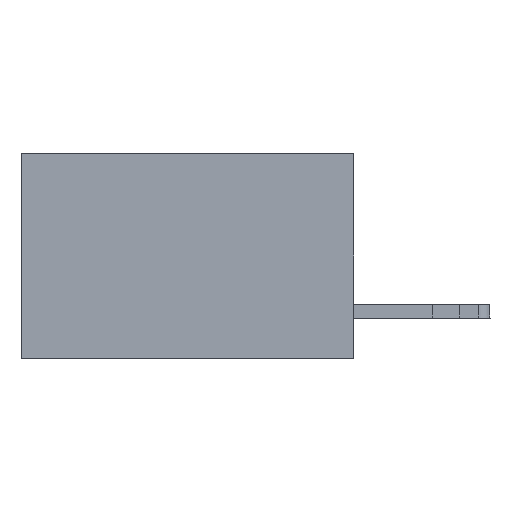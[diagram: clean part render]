
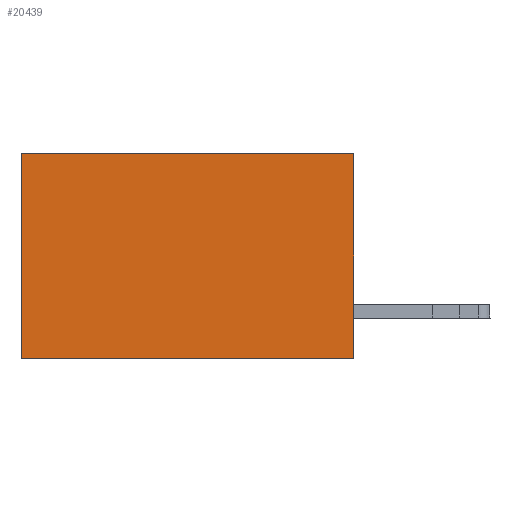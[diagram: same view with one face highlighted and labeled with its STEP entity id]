
A CAD part, left-side view. The second image highlights one B-rep face of the part: STEP entity #20439.
In plain terms, the highlighted planar face has unit normal (-1, 0, 0).
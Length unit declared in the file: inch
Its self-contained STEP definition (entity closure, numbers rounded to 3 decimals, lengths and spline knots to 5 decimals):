
#616 = ORIENTED_EDGE ( 'NONE', *, *, #26338, .T. ) ;
#1786 = VECTOR ( 'NONE', #6886, 39.37008 ) ;
#1950 = VERTEX_POINT ( 'NONE', #5260 ) ;
#3957 = LINE ( 'NONE', #32492, #34746 ) ;
#4269 = DIRECTION ( 'NONE',  ( 0., 1., 0. ) ) ;
#5260 = CARTESIAN_POINT ( 'NONE',  ( 0.2875, 0.6, 0. ) ) ;
#6886 = DIRECTION ( 'NONE',  ( 0., 0., -1. ) ) ;
#7437 = ORIENTED_EDGE ( 'NONE', *, *, #35931, .F. ) ;
#7439 = LINE ( 'NONE', #18447, #1786 ) ;
#8702 = DIRECTION ( 'NONE',  ( 0., 0., -1. ) ) ;
#9938 = VERTEX_POINT ( 'NONE', #36319 ) ;
#10741 = ORIENTED_EDGE ( 'NONE', *, *, #20627, .F. ) ;
#11693 = FACE_OUTER_BOUND ( 'NONE', #29390, .T. ) ;
#11878 = DIRECTION ( 'NONE',  ( 1., 0., 0. ) ) ;
#14487 = CARTESIAN_POINT ( 'NONE',  ( 0.2875, 0., 0. ) ) ;
#14861 = EDGE_CURVE ( 'NONE', #1950, #28969, #7439, .T. ) ;
#15591 = LINE ( 'NONE', #35168, #26474 ) ;
#18447 = CARTESIAN_POINT ( 'NONE',  ( 0.2875, 0.6, 0. ) ) ;
#19942 = PLANE ( 'NONE',  #33562 ) ;
#20439 = ADVANCED_FACE ( 'NONE', ( #11693 ), #19942, .F. ) ;
#20627 = EDGE_CURVE ( 'NONE', #9938, #33087, #15591, .T. ) ;
#21245 = CARTESIAN_POINT ( 'NONE',  ( 0.2875, 0., -0.37 ) ) ;
#21685 = DIRECTION ( 'NONE',  ( 0., 1., 0. ) ) ;
#23055 = CARTESIAN_POINT ( 'NONE',  ( 0.2875, 0., -0.37 ) ) ;
#26338 = EDGE_CURVE ( 'NONE', #9938, #1950, #3957, .T. ) ;
#26474 = VECTOR ( 'NONE', #29604, 39.37008 ) ;
#26479 = VECTOR ( 'NONE', #4269, 39.37008 ) ;
#28969 = VERTEX_POINT ( 'NONE', #34351 ) ;
#29390 = EDGE_LOOP ( 'NONE', ( #35006, #7437, #10741, #616 ) ) ;
#29604 = DIRECTION ( 'NONE',  ( 0., 0., -1. ) ) ;
#32492 = CARTESIAN_POINT ( 'NONE',  ( 0.2875, 0., 0. ) ) ;
#32792 = LINE ( 'NONE', #21245, #26479 ) ;
#33087 = VERTEX_POINT ( 'NONE', #23055 ) ;
#33562 = AXIS2_PLACEMENT_3D ( 'NONE', #14487, #11878, #8702 ) ;
#34351 = CARTESIAN_POINT ( 'NONE',  ( 0.2875, 0.6, -0.37 ) ) ;
#34746 = VECTOR ( 'NONE', #21685, 39.37008 ) ;
#35006 = ORIENTED_EDGE ( 'NONE', *, *, #14861, .T. ) ;
#35168 = CARTESIAN_POINT ( 'NONE',  ( 0.2875, 0., 0. ) ) ;
#35931 = EDGE_CURVE ( 'NONE', #33087, #28969, #32792, .T. ) ;
#36319 = CARTESIAN_POINT ( 'NONE',  ( 0.2875, 0., 0. ) ) ;
